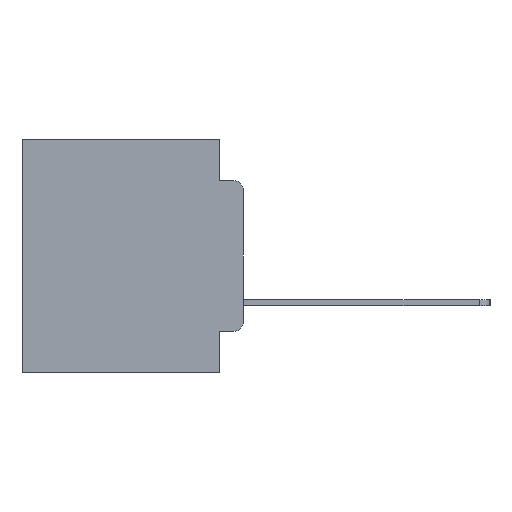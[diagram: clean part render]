
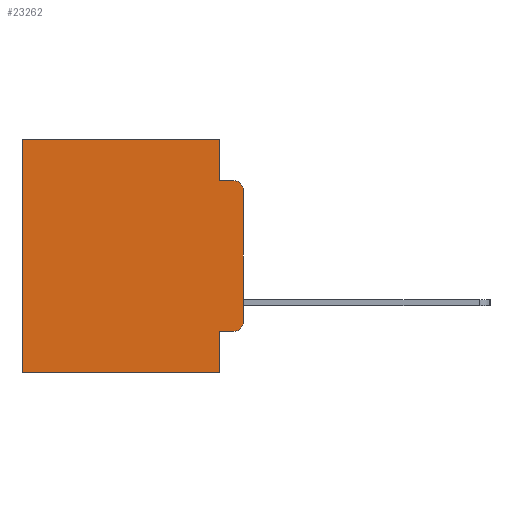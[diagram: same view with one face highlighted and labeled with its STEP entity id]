
A CAD part, left-side view. The second image highlights one B-rep face of the part: STEP entity #23262.
In plain terms, the highlighted planar face has unit normal (-1, 0, 0).
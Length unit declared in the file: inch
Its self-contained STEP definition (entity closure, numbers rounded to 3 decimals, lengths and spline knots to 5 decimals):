
#575 = ORIENTED_EDGE ( 'NONE', *, *, #960, .F. ) ;
#788 = ORIENTED_EDGE ( 'NONE', *, *, #3785, .F. ) ;
#960 = EDGE_CURVE ( 'NONE', #23422, #2283, #23504, .T. ) ;
#1269 = VERTEX_POINT ( 'NONE', #22200 ) ;
#1497 = LINE ( 'NONE', #16074, #12081 ) ;
#1615 = ORIENTED_EDGE ( 'NONE', *, *, #10962, .T. ) ;
#2046 = CARTESIAN_POINT ( 'NONE',  ( 0.298, 0.02, -0.0885 ) ) ;
#2283 = VERTEX_POINT ( 'NONE', #2046 ) ;
#3031 = EDGE_CURVE ( 'NONE', #1269, #5982, #10536, .T. ) ;
#3229 = DIRECTION ( 'NONE',  ( 0., 1., 0. ) ) ;
#3234 = LINE ( 'NONE', #3238, #14313 ) ;
#3238 = CARTESIAN_POINT ( 'NONE',  ( 0.298, 0., -0.5 ) ) ;
#3264 = LINE ( 'NONE', #25902, #8298 ) ;
#3537 = LINE ( 'NONE', #9013, #18682 ) ;
#3785 = EDGE_CURVE ( 'NONE', #20194, #13460, #3234, .T. ) ;
#4482 = DIRECTION ( 'NONE',  ( 0., 0., -1. ) ) ;
#4516 = EDGE_CURVE ( 'NONE', #4749, #1269, #3537, .T. ) ;
#4597 = DIRECTION ( 'NONE',  ( -1., 0., 0. ) ) ;
#4749 = VERTEX_POINT ( 'NONE', #11129 ) ;
#5818 = ORIENTED_EDGE ( 'NONE', *, *, #3031, .T. ) ;
#5982 = VERTEX_POINT ( 'NONE', #6775 ) ;
#6307 = VERTEX_POINT ( 'NONE', #20014 ) ;
#6507 = EDGE_CURVE ( 'NONE', #24928, #6307, #16063, .T. ) ;
#6775 = CARTESIAN_POINT ( 'NONE',  ( 0.298, 0., -0.3915 ) ) ;
#7041 = DIRECTION ( 'NONE',  ( 1., 0., 0. ) ) ;
#7110 = ORIENTED_EDGE ( 'NONE', *, *, #15569, .T. ) ;
#7841 = CARTESIAN_POINT ( 'NONE',  ( 0.298, 0.051, -0.5 ) ) ;
#7887 = FACE_OUTER_BOUND ( 'NONE', #23900, .T. ) ;
#8298 = VECTOR ( 'NONE', #16003, 39.37008 ) ;
#9013 = CARTESIAN_POINT ( 'NONE',  ( 0.298, 0.051, -0.4115 ) ) ;
#9989 = ORIENTED_EDGE ( 'NONE', *, *, #10465, .F. ) ;
#10056 = DIRECTION ( 'NONE',  ( 0., 0., -1. ) ) ;
#10313 = CARTESIAN_POINT ( 'NONE',  ( 0.298, 0.473, -0.5 ) ) ;
#10465 = EDGE_CURVE ( 'NONE', #21599, #5982, #22187, .T. ) ;
#10536 = CIRCLE ( 'NONE', #21735, 0.02 ) ;
#10962 = EDGE_CURVE ( 'NONE', #21599, #2283, #15320, .T. ) ;
#11129 = CARTESIAN_POINT ( 'NONE',  ( 0.298, 0.051, -0.4115 ) ) ;
#11202 = DIRECTION ( 'NONE',  ( 0., 0., -1. ) ) ;
#11462 = EDGE_CURVE ( 'NONE', #4749, #20194, #1497, .T. ) ;
#11760 = ORIENTED_EDGE ( 'NONE', *, *, #6507, .T. ) ;
#12081 = VECTOR ( 'NONE', #10056, 39.37008 ) ;
#12449 = CARTESIAN_POINT ( 'NONE',  ( 0.298, 0.02, -0.1085 ) ) ;
#13460 = VERTEX_POINT ( 'NONE', #10313 ) ;
#13975 = VECTOR ( 'NONE', #14405, 39.37008 ) ;
#14313 = VECTOR ( 'NONE', #3229, 39.37008 ) ;
#14405 = DIRECTION ( 'NONE',  ( 0., 0., -1. ) ) ;
#14507 = DIRECTION ( 'NONE',  ( 0., 0., -1. ) ) ;
#14534 = CARTESIAN_POINT ( 'NONE',  ( 0.298, 0., 0. ) ) ;
#14618 = LINE ( 'NONE', #22375, #13975 ) ;
#15155 = DIRECTION ( 'NONE',  ( 0., -1., 0. ) ) ;
#15320 = CIRCLE ( 'NONE', #20047, 0.02 ) ;
#15439 = VECTOR ( 'NONE', #26465, 39.37008 ) ;
#15569 = EDGE_CURVE ( 'NONE', #6307, #13460, #3264, .T. ) ;
#16003 = DIRECTION ( 'NONE',  ( 0., 0., -1. ) ) ;
#16063 = LINE ( 'NONE', #14534, #15439 ) ;
#16074 = CARTESIAN_POINT ( 'NONE',  ( 0.298, 0.051, 0. ) ) ;
#16923 = EDGE_CURVE ( 'NONE', #24928, #23422, #14618, .T. ) ;
#18199 = CARTESIAN_POINT ( 'NONE',  ( 0.298, 0.051, -0.0885 ) ) ;
#18209 = VECTOR ( 'NONE', #24671, 39.37008 ) ;
#18682 = VECTOR ( 'NONE', #15155, 39.37008 ) ;
#19207 = PLANE ( 'NONE',  #19741 ) ;
#19741 = AXIS2_PLACEMENT_3D ( 'NONE', #25101, #7041, #21208 ) ;
#20014 = CARTESIAN_POINT ( 'NONE',  ( 0.298, 0.473, 0. ) ) ;
#20047 = AXIS2_PLACEMENT_3D ( 'NONE', #12449, #26435, #14507 ) ;
#20194 = VERTEX_POINT ( 'NONE', #7841 ) ;
#21208 = DIRECTION ( 'NONE',  ( 0., 0., -1. ) ) ;
#21402 = ORIENTED_EDGE ( 'NONE', *, *, #11462, .F. ) ;
#21555 = VECTOR ( 'NONE', #11202, 39.37008 ) ;
#21599 = VERTEX_POINT ( 'NONE', #22772 ) ;
#21735 = AXIS2_PLACEMENT_3D ( 'NONE', #22502, #4597, #4482 ) ;
#22187 = LINE ( 'NONE', #23256, #21555 ) ;
#22200 = CARTESIAN_POINT ( 'NONE',  ( 0.298, 0.02, -0.4115 ) ) ;
#22375 = CARTESIAN_POINT ( 'NONE',  ( 0.298, 0.051, 0. ) ) ;
#22502 = CARTESIAN_POINT ( 'NONE',  ( 0.298, 0.02, -0.3915 ) ) ;
#22772 = CARTESIAN_POINT ( 'NONE',  ( 0.298, 0., -0.1085 ) ) ;
#22950 = CARTESIAN_POINT ( 'NONE',  ( 0.298, 0.051, 0. ) ) ;
#23256 = CARTESIAN_POINT ( 'NONE',  ( 0.298, 0., 0. ) ) ;
#23262 = ADVANCED_FACE ( 'NONE', ( #7887 ), #19207, .F. ) ;
#23422 = VERTEX_POINT ( 'NONE', #23818 ) ;
#23504 = LINE ( 'NONE', #18199, #18209 ) ;
#23818 = CARTESIAN_POINT ( 'NONE',  ( 0.298, 0.051, -0.0885 ) ) ;
#23900 = EDGE_LOOP ( 'NONE', ( #9989, #1615, #575, #25589, #11760, #7110, #788, #21402, #23950, #5818 ) ) ;
#23950 = ORIENTED_EDGE ( 'NONE', *, *, #4516, .T. ) ;
#24671 = DIRECTION ( 'NONE',  ( 0., -1., 0. ) ) ;
#24928 = VERTEX_POINT ( 'NONE', #22950 ) ;
#25101 = CARTESIAN_POINT ( 'NONE',  ( 0.298, 0., 0. ) ) ;
#25589 = ORIENTED_EDGE ( 'NONE', *, *, #16923, .F. ) ;
#25902 = CARTESIAN_POINT ( 'NONE',  ( 0.298, 0.473, 0. ) ) ;
#26435 = DIRECTION ( 'NONE',  ( -1., 0., 0. ) ) ;
#26465 = DIRECTION ( 'NONE',  ( 0., 1., 0. ) ) ;
